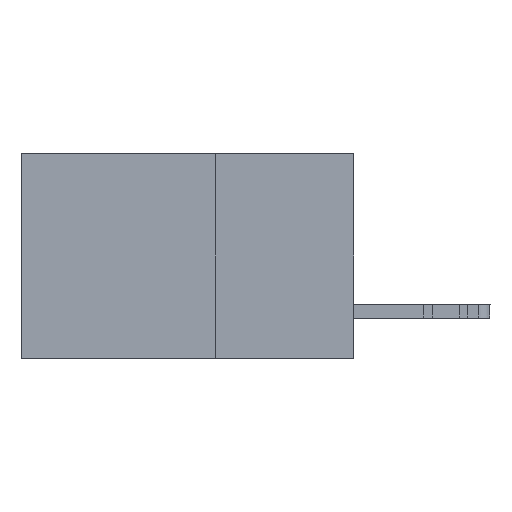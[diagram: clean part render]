
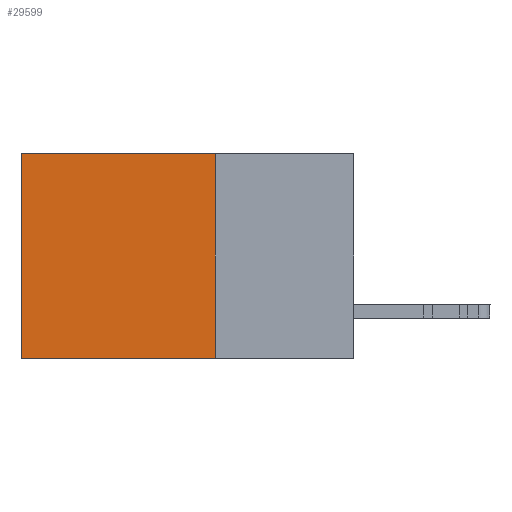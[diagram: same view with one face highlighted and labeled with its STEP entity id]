
A CAD part, left-side view. The second image highlights one B-rep face of the part: STEP entity #29599.
In plain terms, the highlighted planar face has unit normal (-1, 0, 0).
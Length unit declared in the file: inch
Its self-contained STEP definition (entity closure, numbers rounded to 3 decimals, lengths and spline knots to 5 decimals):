
#613 = CARTESIAN_POINT ( 'NONE',  ( 0.2875, 0.6, 0. ) ) ;
#2884 = DIRECTION ( 'NONE',  ( 1., 0., 0. ) ) ;
#4358 = EDGE_LOOP ( 'NONE', ( #39826, #39919, #38590, #43825 ) ) ;
#5750 = CARTESIAN_POINT ( 'NONE',  ( 0.2875, 0.25, 0. ) ) ;
#7238 = VERTEX_POINT ( 'NONE', #29967 ) ;
#10619 = PLANE ( 'NONE',  #41847 ) ;
#10944 = VERTEX_POINT ( 'NONE', #24160 ) ;
#12013 = EDGE_CURVE ( 'NONE', #24168, #10944, #38725, .T. ) ;
#12414 = DIRECTION ( 'NONE',  ( 0., 0., -1. ) ) ;
#12429 = DIRECTION ( 'NONE',  ( 0., 1., 0. ) ) ;
#13602 = CARTESIAN_POINT ( 'NONE',  ( 0.2875, 0.25, 0. ) ) ;
#15250 = CARTESIAN_POINT ( 'NONE',  ( 0.2875, 0.25, 0. ) ) ;
#17619 = EDGE_CURVE ( 'NONE', #7238, #46022, #45398, .T. ) ;
#20106 = LINE ( 'NONE', #23957, #38283 ) ;
#21387 = VECTOR ( 'NONE', #12414, 39.37008 ) ;
#23957 = CARTESIAN_POINT ( 'NONE',  ( 0.2875, 0.25, -0.37 ) ) ;
#24160 = CARTESIAN_POINT ( 'NONE',  ( 0.2875, 0.25, -0.37 ) ) ;
#24168 = VERTEX_POINT ( 'NONE', #15250 ) ;
#25165 = EDGE_CURVE ( 'NONE', #24168, #7238, #35231, .T. ) ;
#28406 = CARTESIAN_POINT ( 'NONE',  ( 0.2875, 0.25, 0. ) ) ;
#29599 = ADVANCED_FACE ( 'NONE', ( #42874 ), #10619, .F. ) ;
#29967 = CARTESIAN_POINT ( 'NONE',  ( 0.2875, 0.6, 0. ) ) ;
#31156 = CARTESIAN_POINT ( 'NONE',  ( 0.2875, 0.6, -0.37 ) ) ;
#33988 = VECTOR ( 'NONE', #35102, 39.37008 ) ;
#35102 = DIRECTION ( 'NONE',  ( 0., 0., -1. ) ) ;
#35231 = LINE ( 'NONE', #13602, #39051 ) ;
#36104 = DIRECTION ( 'NONE',  ( 0., 0., -1. ) ) ;
#36167 = EDGE_CURVE ( 'NONE', #10944, #46022, #20106, .T. ) ;
#38283 = VECTOR ( 'NONE', #12429, 39.37008 ) ;
#38590 = ORIENTED_EDGE ( 'NONE', *, *, #12013, .F. ) ;
#38725 = LINE ( 'NONE', #5750, #33988 ) ;
#38847 = DIRECTION ( 'NONE',  ( 0., 1., 0. ) ) ;
#39051 = VECTOR ( 'NONE', #38847, 39.37008 ) ;
#39826 = ORIENTED_EDGE ( 'NONE', *, *, #17619, .T. ) ;
#39919 = ORIENTED_EDGE ( 'NONE', *, *, #36167, .F. ) ;
#41847 = AXIS2_PLACEMENT_3D ( 'NONE', #28406, #2884, #36104 ) ;
#42874 = FACE_OUTER_BOUND ( 'NONE', #4358, .T. ) ;
#43825 = ORIENTED_EDGE ( 'NONE', *, *, #25165, .T. ) ;
#45398 = LINE ( 'NONE', #613, #21387 ) ;
#46022 = VERTEX_POINT ( 'NONE', #31156 ) ;
